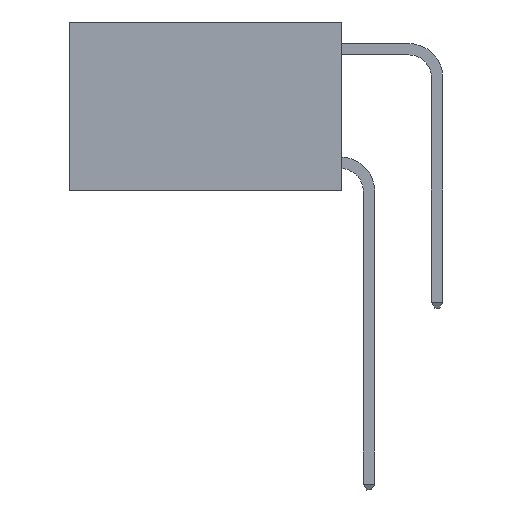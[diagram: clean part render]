
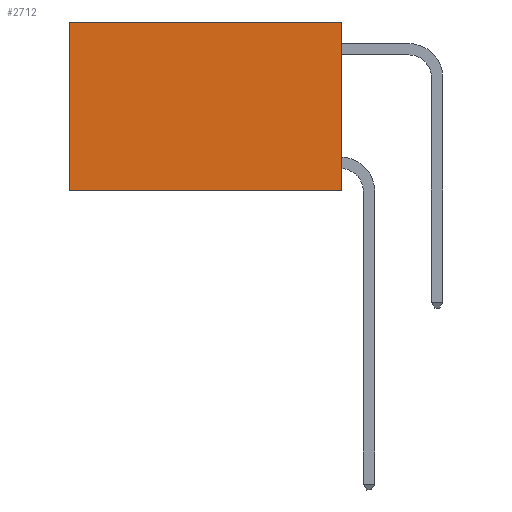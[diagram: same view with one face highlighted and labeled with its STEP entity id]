
A CAD part, left-side view. The second image highlights one B-rep face of the part: STEP entity #2712.
In plain terms, the highlighted planar face has unit normal (-1, 0, 0).
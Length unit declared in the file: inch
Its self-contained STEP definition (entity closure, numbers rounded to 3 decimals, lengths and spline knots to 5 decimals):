
#515 = DIRECTION ( 'NONE',  ( 0., 1., 0. ) ) ;
#594 = CARTESIAN_POINT ( 'NONE',  ( 0.2625, 0., -0.37 ) ) ;
#968 = ORIENTED_EDGE ( 'NONE', *, *, #9022, .F. ) ;
#1512 = CARTESIAN_POINT ( 'NONE',  ( 0.2625, 0., 0. ) ) ;
#1802 = VECTOR ( 'NONE', #15067, 39.37008 ) ;
#1835 = VERTEX_POINT ( 'NONE', #4525 ) ;
#1902 = VERTEX_POINT ( 'NONE', #594 ) ;
#2494 = EDGE_CURVE ( 'NONE', #7199, #1835, #9116, .T. ) ;
#2712 = ADVANCED_FACE ( 'NONE', ( #9603 ), #3251, .F. ) ;
#3167 = EDGE_LOOP ( 'NONE', ( #9079, #968, #8878, #3606 ) ) ;
#3251 = PLANE ( 'NONE',  #3475 ) ;
#3475 = AXIS2_PLACEMENT_3D ( 'NONE', #13281, #14436, #4637 ) ;
#3606 = ORIENTED_EDGE ( 'NONE', *, *, #2494, .T. ) ;
#3887 = CARTESIAN_POINT ( 'NONE',  ( 0.2625, 0., -0.37 ) ) ;
#4525 = CARTESIAN_POINT ( 'NONE',  ( 0.2625, 0.6, 0. ) ) ;
#4631 = CARTESIAN_POINT ( 'NONE',  ( 0.2625, 0.6, -0.37 ) ) ;
#4635 = VECTOR ( 'NONE', #10008, 39.37008 ) ;
#4637 = DIRECTION ( 'NONE',  ( 0., 0., -1. ) ) ;
#5127 = VECTOR ( 'NONE', #9963, 39.37008 ) ;
#6321 = LINE ( 'NONE', #8792, #1802 ) ;
#6467 = LINE ( 'NONE', #3887, #4635 ) ;
#7199 = VERTEX_POINT ( 'NONE', #11358 ) ;
#8792 = CARTESIAN_POINT ( 'NONE',  ( 0.2625, 0.6, 0. ) ) ;
#8878 = ORIENTED_EDGE ( 'NONE', *, *, #8904, .F. ) ;
#8904 = EDGE_CURVE ( 'NONE', #7199, #1902, #11583, .T. ) ;
#9022 = EDGE_CURVE ( 'NONE', #1902, #15049, #6467, .T. ) ;
#9079 = ORIENTED_EDGE ( 'NONE', *, *, #10969, .T. ) ;
#9116 = LINE ( 'NONE', #12955, #12495 ) ;
#9603 = FACE_OUTER_BOUND ( 'NONE', #3167, .T. ) ;
#9963 = DIRECTION ( 'NONE',  ( 0., 0., -1. ) ) ;
#10008 = DIRECTION ( 'NONE',  ( 0., 1., 0. ) ) ;
#10969 = EDGE_CURVE ( 'NONE', #1835, #15049, #6321, .T. ) ;
#11358 = CARTESIAN_POINT ( 'NONE',  ( 0.2625, 0., 0. ) ) ;
#11583 = LINE ( 'NONE', #1512, #5127 ) ;
#12495 = VECTOR ( 'NONE', #515, 39.37008 ) ;
#12955 = CARTESIAN_POINT ( 'NONE',  ( 0.2625, 0., 0. ) ) ;
#13281 = CARTESIAN_POINT ( 'NONE',  ( 0.2625, 0., 0. ) ) ;
#14436 = DIRECTION ( 'NONE',  ( 1., 0., 0. ) ) ;
#15049 = VERTEX_POINT ( 'NONE', #4631 ) ;
#15067 = DIRECTION ( 'NONE',  ( 0., 0., -1. ) ) ;
